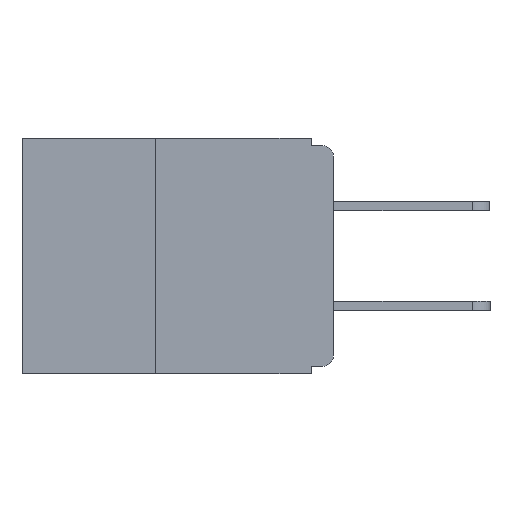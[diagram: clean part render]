
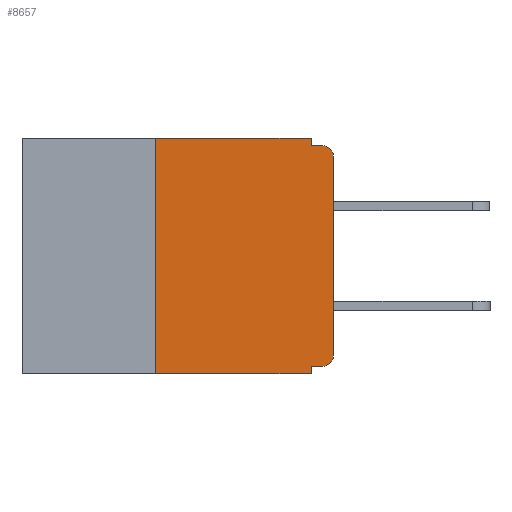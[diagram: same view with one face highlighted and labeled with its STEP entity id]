
A CAD part, left-side view. The second image highlights one B-rep face of the part: STEP entity #8657.
In plain terms, the highlighted planar face has unit normal (-1, 0, 0).
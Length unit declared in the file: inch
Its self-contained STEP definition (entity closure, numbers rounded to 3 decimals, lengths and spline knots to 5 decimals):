
#26 = CARTESIAN_POINT ( 'NONE',  ( 0., 0.25, -0.33 ) ) ;
#574 = CARTESIAN_POINT ( 'NONE',  ( 0., 0.437, 0. ) ) ;
#921 = LINE ( 'NONE', #574, #17522 ) ;
#1044 = VERTEX_POINT ( 'NONE', #21014 ) ;
#1314 = CARTESIAN_POINT ( 'NONE',  ( 0., 0.015, -0.32 ) ) ;
#1679 = DIRECTION ( 'NONE',  ( 0., -1., 0. ) ) ;
#1744 = CARTESIAN_POINT ( 'NONE',  ( 0., 0., 0. ) ) ;
#1954 = VERTEX_POINT ( 'NONE', #13756 ) ;
#2050 = VERTEX_POINT ( 'NONE', #11160 ) ;
#2342 = DIRECTION ( 'NONE',  ( 0., -1., 0. ) ) ;
#2531 = VERTEX_POINT ( 'NONE', #1314 ) ;
#2569 = CARTESIAN_POINT ( 'NONE',  ( 0., 0.031, 0. ) ) ;
#3573 = DIRECTION ( 'NONE',  ( 0., 0., 1. ) ) ;
#4297 = DIRECTION ( 'NONE',  ( 0., 1., 0. ) ) ;
#4359 = EDGE_CURVE ( 'NONE', #10022, #2050, #7571, .T. ) ;
#4890 = CARTESIAN_POINT ( 'NONE',  ( 0., 0., -0.025 ) ) ;
#5773 = CARTESIAN_POINT ( 'NONE',  ( 0., 0.031, -0.33 ) ) ;
#6257 = VECTOR ( 'NONE', #14894, 39.37008 ) ;
#6519 = ORIENTED_EDGE ( 'NONE', *, *, #15706, .T. ) ;
#6823 = CARTESIAN_POINT ( 'NONE',  ( 0., 0.437, -0.33 ) ) ;
#6889 = DIRECTION ( 'NONE',  ( 0., 0., 1. ) ) ;
#7323 = DIRECTION ( 'NONE',  ( -1., 0., 0. ) ) ;
#7350 = LINE ( 'NONE', #19693, #6257 ) ;
#7490 = DIRECTION ( 'NONE',  ( 0., 0., -1. ) ) ;
#7537 = DIRECTION ( 'NONE',  ( -1., 0., 0. ) ) ;
#7571 = LINE ( 'NONE', #10394, #19873 ) ;
#7588 = ORIENTED_EDGE ( 'NONE', *, *, #17754, .F. ) ;
#8110 = VERTEX_POINT ( 'NONE', #19750 ) ;
#8430 = ORIENTED_EDGE ( 'NONE', *, *, #19940, .F. ) ;
#8500 = VECTOR ( 'NONE', #6889, 39.37008 ) ;
#8531 = ORIENTED_EDGE ( 'NONE', *, *, #4359, .F. ) ;
#8657 = ADVANCED_FACE ( 'NONE', ( #19964 ), #21415, .F. ) ;
#8982 = VERTEX_POINT ( 'NONE', #15958 ) ;
#9349 = CARTESIAN_POINT ( 'NONE',  ( 0., 0., -0.32 ) ) ;
#9362 = CIRCLE ( 'NONE', #17088, 0.015 ) ;
#9784 = ORIENTED_EDGE ( 'NONE', *, *, #16396, .F. ) ;
#10022 = VERTEX_POINT ( 'NONE', #2569 ) ;
#10394 = CARTESIAN_POINT ( 'NONE',  ( 0., 0.031, 0. ) ) ;
#10733 = CARTESIAN_POINT ( 'NONE',  ( 0., 0.031, -0.33 ) ) ;
#10806 = DIRECTION ( 'NONE',  ( 0., 0., -1. ) ) ;
#10840 = ORIENTED_EDGE ( 'NONE', *, *, #11150, .T. ) ;
#11150 = EDGE_CURVE ( 'NONE', #2531, #1044, #11877, .T. ) ;
#11160 = CARTESIAN_POINT ( 'NONE',  ( 0., 0.031, -0.01 ) ) ;
#11336 = ORIENTED_EDGE ( 'NONE', *, *, #16874, .F. ) ;
#11877 = CIRCLE ( 'NONE', #17028, 0.015 ) ;
#12005 = EDGE_LOOP ( 'NONE', ( #19319, #6519, #7588, #8531, #9784, #11336, #19904, #8430, #14695, #10840 ) ) ;
#12190 = EDGE_CURVE ( 'NONE', #1044, #13220, #21755, .T. ) ;
#12247 = LINE ( 'NONE', #5773, #20930 ) ;
#13220 = VERTEX_POINT ( 'NONE', #4890 ) ;
#13680 = VECTOR ( 'NONE', #3573, 39.37008 ) ;
#13756 = CARTESIAN_POINT ( 'NONE',  ( 0., 0.031, -0.32 ) ) ;
#13973 = AXIS2_PLACEMENT_3D ( 'NONE', #20897, #21348, #17249 ) ;
#14442 = VERTEX_POINT ( 'NONE', #15696 ) ;
#14695 = ORIENTED_EDGE ( 'NONE', *, *, #21090, .F. ) ;
#14894 = DIRECTION ( 'NONE',  ( 0., -1., 0. ) ) ;
#15696 = CARTESIAN_POINT ( 'NONE',  ( 0., 0.015, -0.01 ) ) ;
#15706 = EDGE_CURVE ( 'NONE', #13220, #14442, #9362, .T. ) ;
#15891 = VECTOR ( 'NONE', #1679, 39.37008 ) ;
#15958 = CARTESIAN_POINT ( 'NONE',  ( 0., 0.25, 0. ) ) ;
#16396 = EDGE_CURVE ( 'NONE', #8982, #10022, #921, .T. ) ;
#16874 = EDGE_CURVE ( 'NONE', #8110, #8982, #17973, .T. ) ;
#17028 = AXIS2_PLACEMENT_3D ( 'NONE', #17688, #7537, #19269 ) ;
#17088 = AXIS2_PLACEMENT_3D ( 'NONE', #17503, #7323, #19087 ) ;
#17217 = VECTOR ( 'NONE', #4297, 39.37008 ) ;
#17249 = DIRECTION ( 'NONE',  ( 0., 0., -1. ) ) ;
#17503 = CARTESIAN_POINT ( 'NONE',  ( 0., 0.015, -0.025 ) ) ;
#17522 = VECTOR ( 'NONE', #2342, 39.37008 ) ;
#17688 = CARTESIAN_POINT ( 'NONE',  ( 0., 0.015, -0.305 ) ) ;
#17700 = LINE ( 'NONE', #9349, #17217 ) ;
#17754 = EDGE_CURVE ( 'NONE', #2050, #14442, #7350, .T. ) ;
#17973 = LINE ( 'NONE', #26, #8500 ) ;
#18583 = EDGE_CURVE ( 'NONE', #8110, #20472, #20125, .T. ) ;
#19087 = DIRECTION ( 'NONE',  ( 0., 0., -1. ) ) ;
#19269 = DIRECTION ( 'NONE',  ( 0., 0., -1. ) ) ;
#19319 = ORIENTED_EDGE ( 'NONE', *, *, #12190, .T. ) ;
#19693 = CARTESIAN_POINT ( 'NONE',  ( 0., 0., -0.01 ) ) ;
#19750 = CARTESIAN_POINT ( 'NONE',  ( 0., 0.25, -0.33 ) ) ;
#19873 = VECTOR ( 'NONE', #10806, 39.37008 ) ;
#19904 = ORIENTED_EDGE ( 'NONE', *, *, #18583, .T. ) ;
#19940 = EDGE_CURVE ( 'NONE', #1954, #20472, #12247, .T. ) ;
#19964 = FACE_OUTER_BOUND ( 'NONE', #12005, .T. ) ;
#20125 = LINE ( 'NONE', #6823, #15891 ) ;
#20472 = VERTEX_POINT ( 'NONE', #10733 ) ;
#20897 = CARTESIAN_POINT ( 'NONE',  ( 0., 0.437, 0. ) ) ;
#20930 = VECTOR ( 'NONE', #7490, 39.37008 ) ;
#21014 = CARTESIAN_POINT ( 'NONE',  ( 0., 0., -0.305 ) ) ;
#21090 = EDGE_CURVE ( 'NONE', #2531, #1954, #17700, .T. ) ;
#21348 = DIRECTION ( 'NONE',  ( 1., 0., 0. ) ) ;
#21415 = PLANE ( 'NONE',  #13973 ) ;
#21755 = LINE ( 'NONE', #1744, #13680 ) ;
